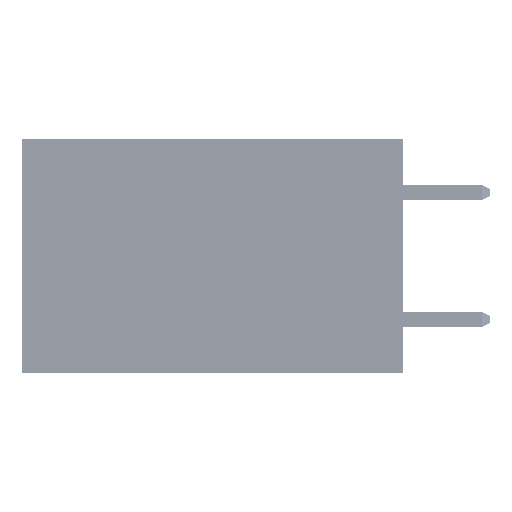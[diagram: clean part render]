
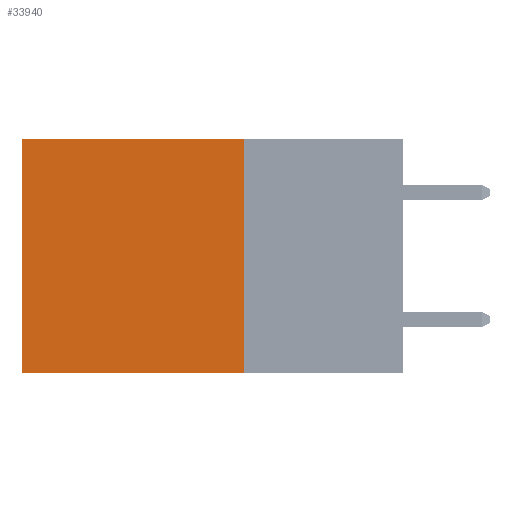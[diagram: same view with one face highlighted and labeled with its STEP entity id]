
A CAD part, left-side view. The second image highlights one B-rep face of the part: STEP entity #33940.
In plain terms, the highlighted planar face has unit normal (-1, 0, 0).
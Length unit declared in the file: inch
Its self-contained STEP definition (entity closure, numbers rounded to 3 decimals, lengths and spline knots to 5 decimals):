
#1214 = LINE ( 'NONE', #35877, #20514 ) ;
#1301 = ORIENTED_EDGE ( 'NONE', *, *, #48300, .T. ) ;
#4338 = EDGE_CURVE ( 'NONE', #34614, #22023, #40520, .T. ) ;
#7000 = VECTOR ( 'NONE', #48707, 39.37008 ) ;
#7862 = LINE ( 'NONE', #16819, #42119 ) ;
#8292 = DIRECTION ( 'NONE',  ( 0., 1., 0. ) ) ;
#11159 = FACE_OUTER_BOUND ( 'NONE', #16825, .T. ) ;
#12428 = DIRECTION ( 'NONE',  ( 0., 0., -1. ) ) ;
#12594 = DIRECTION ( 'NONE',  ( 1., 0., 0. ) ) ;
#16072 = VERTEX_POINT ( 'NONE', #28367 ) ;
#16293 = CARTESIAN_POINT ( 'NONE',  ( 0.2875, 0.25, 0. ) ) ;
#16819 = CARTESIAN_POINT ( 'NONE',  ( 0.2875, 0.6, 0. ) ) ;
#16825 = EDGE_LOOP ( 'NONE', ( #1301, #22414, #33082, #28994 ) ) ;
#17666 = EDGE_CURVE ( 'NONE', #45961, #34614, #19671, .T. ) ;
#18291 = VECTOR ( 'NONE', #8292, 39.37008 ) ;
#19671 = LINE ( 'NONE', #30091, #7000 ) ;
#19841 = PLANE ( 'NONE',  #42468 ) ;
#20514 = VECTOR ( 'NONE', #39067, 39.37008 ) ;
#20800 = CARTESIAN_POINT ( 'NONE',  ( 0.2875, 0.6, -0.37 ) ) ;
#21906 = EDGE_CURVE ( 'NONE', #45961, #16072, #1214, .T. ) ;
#22023 = VERTEX_POINT ( 'NONE', #20800 ) ;
#22414 = ORIENTED_EDGE ( 'NONE', *, *, #4338, .F. ) ;
#27739 = CARTESIAN_POINT ( 'NONE',  ( 0.2875, 0.25, 0. ) ) ;
#28367 = CARTESIAN_POINT ( 'NONE',  ( 0.2875, 0.6, 0. ) ) ;
#28994 = ORIENTED_EDGE ( 'NONE', *, *, #21906, .T. ) ;
#30091 = CARTESIAN_POINT ( 'NONE',  ( 0.2875, 0.25, 0. ) ) ;
#31443 = DIRECTION ( 'NONE',  ( 0., 0., -1. ) ) ;
#33082 = ORIENTED_EDGE ( 'NONE', *, *, #17666, .F. ) ;
#33940 = ADVANCED_FACE ( 'NONE', ( #11159 ), #19841, .F. ) ;
#34614 = VERTEX_POINT ( 'NONE', #47275 ) ;
#35877 = CARTESIAN_POINT ( 'NONE',  ( 0.2875, 0.25, 0. ) ) ;
#39067 = DIRECTION ( 'NONE',  ( 0., 1., 0. ) ) ;
#40520 = LINE ( 'NONE', #43350, #18291 ) ;
#42119 = VECTOR ( 'NONE', #31443, 39.37008 ) ;
#42468 = AXIS2_PLACEMENT_3D ( 'NONE', #27739, #12594, #12428 ) ;
#43350 = CARTESIAN_POINT ( 'NONE',  ( 0.2875, 0.25, -0.37 ) ) ;
#45961 = VERTEX_POINT ( 'NONE', #16293 ) ;
#47275 = CARTESIAN_POINT ( 'NONE',  ( 0.2875, 0.25, -0.37 ) ) ;
#48300 = EDGE_CURVE ( 'NONE', #16072, #22023, #7862, .T. ) ;
#48707 = DIRECTION ( 'NONE',  ( 0., 0., -1. ) ) ;
